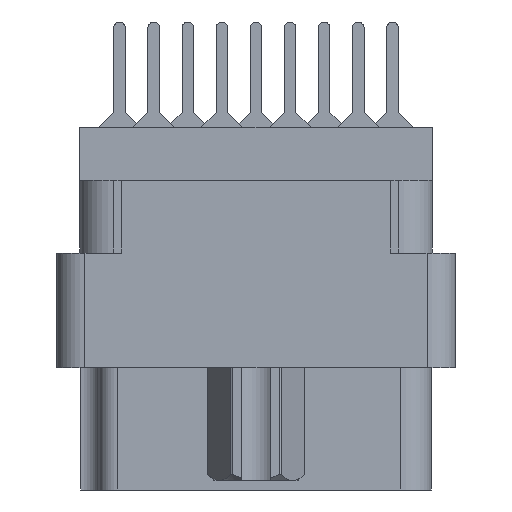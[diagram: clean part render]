
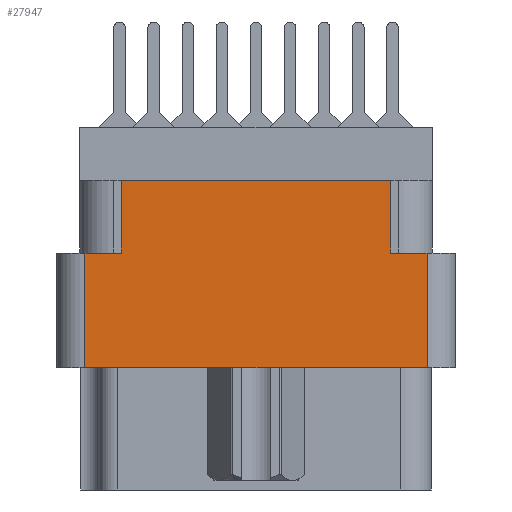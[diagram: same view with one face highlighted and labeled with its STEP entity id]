
A CAD part, left-side view. The second image highlights one B-rep face of the part: STEP entity #27947.
In plain terms, the highlighted planar face has unit normal (-1, 0, 0).
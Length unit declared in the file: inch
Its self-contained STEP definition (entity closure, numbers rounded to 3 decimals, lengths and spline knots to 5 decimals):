
#274 = ORIENTED_EDGE ( 'NONE', *, *, #7468, .T. ) ;
#309 = EDGE_CURVE ( 'NONE', #43970, #46058, #37545, .T. ) ;
#329 = CARTESIAN_POINT ( 'NONE',  ( -1., -0.296, -0.277 ) ) ;
#792 = LINE ( 'NONE', #21359, #9352 ) ;
#2229 = DIRECTION ( 'NONE',  ( 0., 1., 0. ) ) ;
#3490 = EDGE_CURVE ( 'NONE', #33060, #29408, #20747, .T. ) ;
#5156 = VECTOR ( 'NONE', #40752, 39.37008 ) ;
#6274 = VERTEX_POINT ( 'NONE', #14665 ) ;
#7468 = EDGE_CURVE ( 'NONE', #29651, #46058, #26313, .T. ) ;
#8106 = VECTOR ( 'NONE', #8955, 39.37008 ) ;
#8955 = DIRECTION ( 'NONE',  ( 0., -1., 0. ) ) ;
#9352 = VECTOR ( 'NONE', #17823, 39.37008 ) ;
#9404 = ORIENTED_EDGE ( 'NONE', *, *, #44997, .F. ) ;
#10351 = CARTESIAN_POINT ( 'NONE',  ( -1., 0.296, -0.277 ) ) ;
#12462 = CARTESIAN_POINT ( 'NONE',  ( -1., 0.376, -0.529 ) ) ;
#12480 = CARTESIAN_POINT ( 'NONE',  ( -1., 0.296, -0.117 ) ) ;
#13420 = CARTESIAN_POINT ( 'NONE',  ( -1., -0.376, -0.529 ) ) ;
#13526 = DIRECTION ( 'NONE',  ( 0., 0., 1. ) ) ;
#13569 = AXIS2_PLACEMENT_3D ( 'NONE', #42463, #39033, #13526 ) ;
#13683 = ORIENTED_EDGE ( 'NONE', *, *, #309, .F. ) ;
#13687 = EDGE_CURVE ( 'NONE', #29651, #37632, #792, .T. ) ;
#13926 = CARTESIAN_POINT ( 'NONE',  ( -1., -0.376, -0.798 ) ) ;
#14665 = CARTESIAN_POINT ( 'NONE',  ( -1., -0.376, -0.277 ) ) ;
#16560 = VECTOR ( 'NONE', #40406, 39.37008 ) ;
#17823 = DIRECTION ( 'NONE',  ( 0., -1., 0. ) ) ;
#17841 = CARTESIAN_POINT ( 'NONE',  ( -1., 0.376, -0.798 ) ) ;
#18538 = LINE ( 'NONE', #25237, #32254 ) ;
#18937 = CARTESIAN_POINT ( 'NONE',  ( -1., 0.376, -0.277 ) ) ;
#20313 = CARTESIAN_POINT ( 'NONE',  ( -1., 0., -0.277 ) ) ;
#20747 = LINE ( 'NONE', #329, #5156 ) ;
#21359 = CARTESIAN_POINT ( 'NONE',  ( -1., 0., -0.277 ) ) ;
#23240 = ORIENTED_EDGE ( 'NONE', *, *, #31040, .F. ) ;
#23411 = ORIENTED_EDGE ( 'NONE', *, *, #36386, .T. ) ;
#23543 = VERTEX_POINT ( 'NONE', #12480 ) ;
#23984 = DIRECTION ( 'NONE',  ( 0., -1., 0. ) ) ;
#25005 = DIRECTION ( 'NONE',  ( 0., 0., 1. ) ) ;
#25006 = CARTESIAN_POINT ( 'NONE',  ( -1., -0.296, -0.117 ) ) ;
#25237 = CARTESIAN_POINT ( 'NONE',  ( -1., 0.296, -0.277 ) ) ;
#25485 = VECTOR ( 'NONE', #2229, 39.37008 ) ;
#25647 = FACE_OUTER_BOUND ( 'NONE', #34017, .T. ) ;
#25926 = LINE ( 'NONE', #45575, #8106 ) ;
#26313 = LINE ( 'NONE', #17841, #16560 ) ;
#27654 = PLANE ( 'NONE',  #13569 ) ;
#27658 = VECTOR ( 'NONE', #25005, 39.37008 ) ;
#27896 = ORIENTED_EDGE ( 'NONE', *, *, #33734, .F. ) ;
#27947 = ADVANCED_FACE ( 'NONE', ( #25647 ), #27654, .T. ) ;
#28253 = LINE ( 'NONE', #13926, #27658 ) ;
#29408 = VERTEX_POINT ( 'NONE', #25006 ) ;
#29651 = VERTEX_POINT ( 'NONE', #18937 ) ;
#30652 = VECTOR ( 'NONE', #23984, 39.37008 ) ;
#30759 = CARTESIAN_POINT ( 'NONE',  ( -1., 0., -0.529 ) ) ;
#31040 = EDGE_CURVE ( 'NONE', #23543, #29408, #25926, .T. ) ;
#32254 = VECTOR ( 'NONE', #39984, 39.37008 ) ;
#33060 = VERTEX_POINT ( 'NONE', #41836 ) ;
#33734 = EDGE_CURVE ( 'NONE', #33060, #6274, #36143, .T. ) ;
#34017 = EDGE_LOOP ( 'NONE', ( #40581, #274, #13683, #23411, #27896, #37422, #23240, #9404 ) ) ;
#36143 = LINE ( 'NONE', #20313, #30652 ) ;
#36386 = EDGE_CURVE ( 'NONE', #43970, #6274, #28253, .T. ) ;
#37422 = ORIENTED_EDGE ( 'NONE', *, *, #3490, .T. ) ;
#37545 = LINE ( 'NONE', #30759, #25485 ) ;
#37632 = VERTEX_POINT ( 'NONE', #10351 ) ;
#39033 = DIRECTION ( 'NONE',  ( -1., 0., 0. ) ) ;
#39984 = DIRECTION ( 'NONE',  ( 0., 0., 1. ) ) ;
#40406 = DIRECTION ( 'NONE',  ( 0., 0., -1. ) ) ;
#40581 = ORIENTED_EDGE ( 'NONE', *, *, #13687, .F. ) ;
#40752 = DIRECTION ( 'NONE',  ( 0., 0., 1. ) ) ;
#41836 = CARTESIAN_POINT ( 'NONE',  ( -1., -0.296, -0.277 ) ) ;
#42463 = CARTESIAN_POINT ( 'NONE',  ( -1., -0.438, -0.798 ) ) ;
#43970 = VERTEX_POINT ( 'NONE', #13420 ) ;
#44997 = EDGE_CURVE ( 'NONE', #37632, #23543, #18538, .T. ) ;
#45575 = CARTESIAN_POINT ( 'NONE',  ( -1., 0.438, -0.117 ) ) ;
#46058 = VERTEX_POINT ( 'NONE', #12462 ) ;
